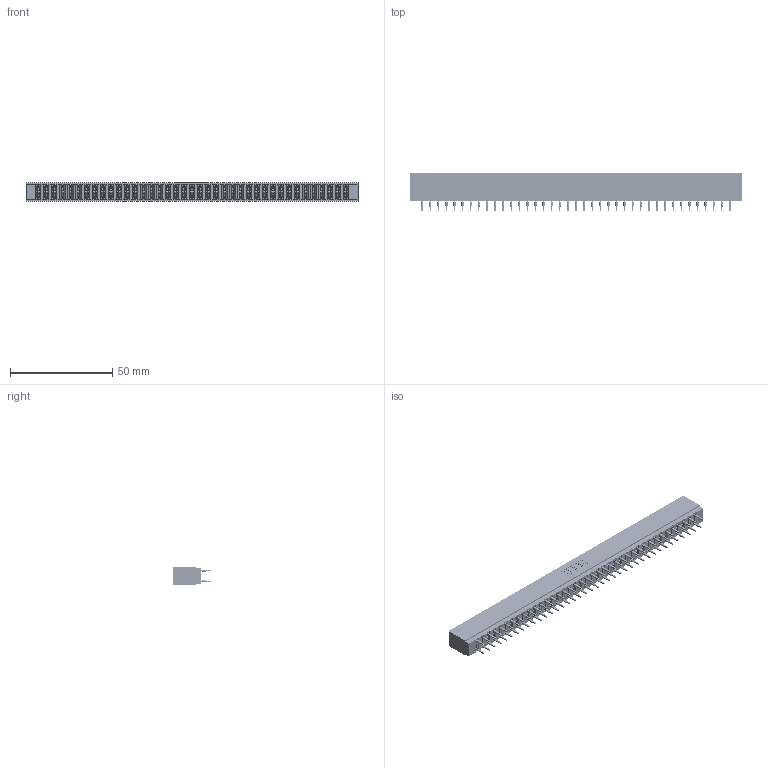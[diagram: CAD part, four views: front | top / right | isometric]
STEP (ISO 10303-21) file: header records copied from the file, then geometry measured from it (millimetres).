
FILE_DESCRIPTION (( 'STEP AP203' ), '1' );
FILE_NAME ('717-078-560-201.STEP', '2026-02-20T19:24:47', ( '' ), ( '' ), 'SwSTEP 2.0', 'SolidWorks 2023', '' );
FILE_SCHEMA (( 'CONFIG_CONTROL_DESIGN' ));
Length unit declared in the file: millimetre
Products named in the file (3): 745-292-001_560; 717 Part_Insulator Option - 06; 717-078-560-201
Assembly tree (79 placements, depth 2):
  717-078-560-201
    717 Part_Insulator Option - 06
    745-292-001_560  x78
Bounding box: 162.41 x 18.78 x 8.89 mm (x, y, z)
Volume: 14373.2 mm3; surface area: 23319.6 mm2
Topology: 79 solids, 79 shells, 7816 faces, 21389 edges, 13582 vertices
Faces by surface type: plane 4071, cylinder 1717, bspline 1560, torus 468
Entity records: 67608 total; most frequent: CARTESIAN_POINT 12241, ORIENTED_EDGE 11670, DIRECTION 10195, EDGE_CURVE 5835, VECTOR 5411, LINE 5411, VERTEX_POINT 3726, AXIS2_PLACEMENT_3D 2392
